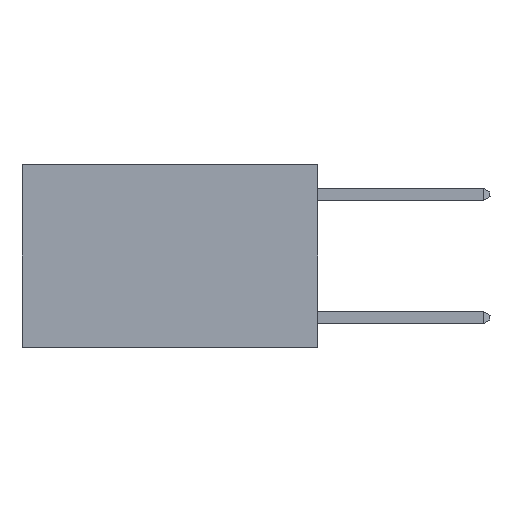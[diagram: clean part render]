
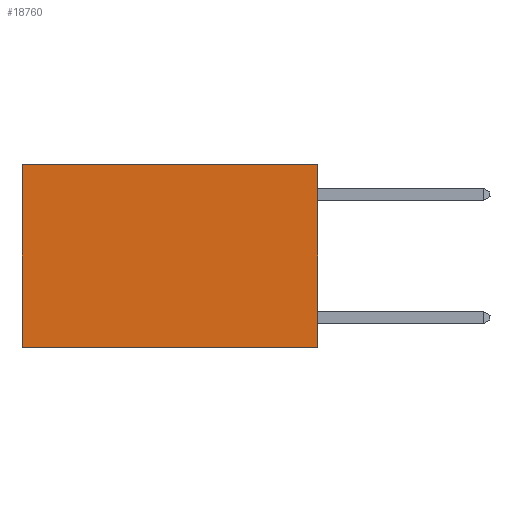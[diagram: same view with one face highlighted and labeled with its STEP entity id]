
A CAD part, left-side view. The second image highlights one B-rep face of the part: STEP entity #18760.
In plain terms, the highlighted planar face has unit normal (-1, 0, 0).
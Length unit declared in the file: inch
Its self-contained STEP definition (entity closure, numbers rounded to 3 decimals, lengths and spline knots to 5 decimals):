
#78 = FACE_OUTER_BOUND ( 'NONE', #10549, .T. ) ;
#2564 = ORIENTED_EDGE ( 'NONE', *, *, #10376, .F. ) ;
#3382 = CARTESIAN_POINT ( 'NONE',  ( 0.2625, 0.6, 0. ) ) ;
#3708 = LINE ( 'NONE', #23468, #21997 ) ;
#4865 = VERTEX_POINT ( 'NONE', #11268 ) ;
#5935 = CARTESIAN_POINT ( 'NONE',  ( 0.2625, 0., -0.37 ) ) ;
#8571 = CARTESIAN_POINT ( 'NONE',  ( 0.2625, 0.6, 0. ) ) ;
#10376 = EDGE_CURVE ( 'NONE', #14247, #4865, #12707, .T. ) ;
#10549 = EDGE_LOOP ( 'NONE', ( #13326, #2564, #21655, #24646 ) ) ;
#10851 = DIRECTION ( 'NONE',  ( 0., 0., -1. ) ) ;
#11268 = CARTESIAN_POINT ( 'NONE',  ( 0.2625, 0.6, -0.37 ) ) ;
#12399 = CARTESIAN_POINT ( 'NONE',  ( 0.2625, 0., 0. ) ) ;
#12679 = EDGE_CURVE ( 'NONE', #28110, #4865, #20744, .T. ) ;
#12707 = LINE ( 'NONE', #26889, #13062 ) ;
#13062 = VECTOR ( 'NONE', #15337, 39.37008 ) ;
#13326 = ORIENTED_EDGE ( 'NONE', *, *, #12679, .T. ) ;
#14247 = VERTEX_POINT ( 'NONE', #5935 ) ;
#14335 = AXIS2_PLACEMENT_3D ( 'NONE', #12399, #29399, #19679 ) ;
#15289 = CARTESIAN_POINT ( 'NONE',  ( 0.2625, 0., 0. ) ) ;
#15337 = DIRECTION ( 'NONE',  ( 0., 1., 0. ) ) ;
#17616 = EDGE_CURVE ( 'NONE', #20777, #14247, #28982, .T. ) ;
#18760 = ADVANCED_FACE ( 'NONE', ( #78 ), #21120, .F. ) ;
#18944 = VECTOR ( 'NONE', #10851, 39.37008 ) ;
#19679 = DIRECTION ( 'NONE',  ( 0., 0., -1. ) ) ;
#20481 = DIRECTION ( 'NONE',  ( 0., 0., -1. ) ) ;
#20744 = LINE ( 'NONE', #8571, #24782 ) ;
#20777 = VERTEX_POINT ( 'NONE', #29853 ) ;
#21120 = PLANE ( 'NONE',  #14335 ) ;
#21242 = DIRECTION ( 'NONE',  ( 0., 1., 0. ) ) ;
#21655 = ORIENTED_EDGE ( 'NONE', *, *, #17616, .F. ) ;
#21997 = VECTOR ( 'NONE', #21242, 39.37008 ) ;
#23468 = CARTESIAN_POINT ( 'NONE',  ( 0.2625, 0., 0. ) ) ;
#24646 = ORIENTED_EDGE ( 'NONE', *, *, #25881, .T. ) ;
#24782 = VECTOR ( 'NONE', #20481, 39.37008 ) ;
#25881 = EDGE_CURVE ( 'NONE', #20777, #28110, #3708, .T. ) ;
#26889 = CARTESIAN_POINT ( 'NONE',  ( 0.2625, 0., -0.37 ) ) ;
#28110 = VERTEX_POINT ( 'NONE', #3382 ) ;
#28982 = LINE ( 'NONE', #15289, #18944 ) ;
#29399 = DIRECTION ( 'NONE',  ( 1., 0., 0. ) ) ;
#29853 = CARTESIAN_POINT ( 'NONE',  ( 0.2625, 0., 0. ) ) ;
